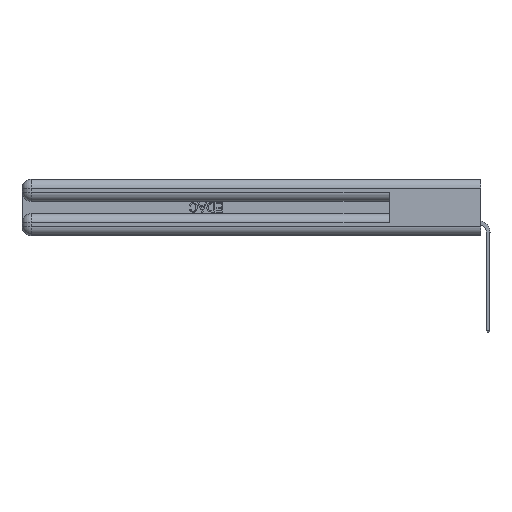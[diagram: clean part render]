
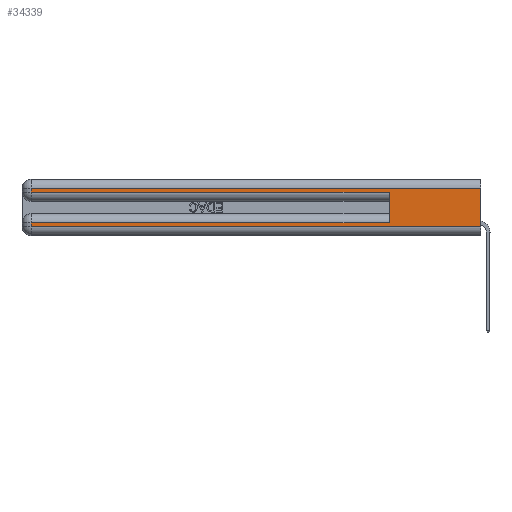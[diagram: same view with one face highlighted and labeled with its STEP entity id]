
A CAD part, left-side view. The second image highlights one B-rep face of the part: STEP entity #34339.
In plain terms, the highlighted planar face has unit normal (-1, 0, 0).
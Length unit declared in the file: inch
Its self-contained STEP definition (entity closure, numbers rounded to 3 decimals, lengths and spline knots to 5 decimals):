
#179 = VECTOR ( 'NONE', #30480, 39.37008 ) ;
#824 = CARTESIAN_POINT ( 'NONE',  ( 0., 2.94, 0.37 ) ) ;
#914 = CARTESIAN_POINT ( 'NONE',  ( 0., 0.6, 0.085 ) ) ;
#1664 = CARTESIAN_POINT ( 'NONE',  ( 0., 0., 0.31 ) ) ;
#2290 = EDGE_CURVE ( 'NONE', #16596, #33285, #25107, .T. ) ;
#2438 = VECTOR ( 'NONE', #9605, 39.37008 ) ;
#3747 = LINE ( 'NONE', #824, #2438 ) ;
#3851 = CARTESIAN_POINT ( 'NONE',  ( 0., 2.94, 0.37 ) ) ;
#4039 = DIRECTION ( 'NONE',  ( 0., 0., -1. ) ) ;
#4393 = FACE_OUTER_BOUND ( 'NONE', #9699, .T. ) ;
#5844 = ORIENTED_EDGE ( 'NONE', *, *, #26525, .F. ) ;
#5967 = CARTESIAN_POINT ( 'NONE',  ( 0., 2.94, 0.285 ) ) ;
#6519 = VERTEX_POINT ( 'NONE', #26959 ) ;
#6726 = DIRECTION ( 'NONE',  ( 0., 0., -1. ) ) ;
#8033 = CARTESIAN_POINT ( 'NONE',  ( 0., 2.94, 0.31 ) ) ;
#8078 = VECTOR ( 'NONE', #27937, 39.37008 ) ;
#8885 = ORIENTED_EDGE ( 'NONE', *, *, #13272, .T. ) ;
#9605 = DIRECTION ( 'NONE',  ( 0., 0., -1. ) ) ;
#9699 = EDGE_LOOP ( 'NONE', ( #5844, #21100, #18361, #8885, #35085, #35553, #29935, #29066 ) ) ;
#10263 = VERTEX_POINT ( 'NONE', #914 ) ;
#10519 = VERTEX_POINT ( 'NONE', #1664 ) ;
#11010 = EDGE_CURVE ( 'NONE', #10519, #34009, #36066, .T. ) ;
#12023 = CARTESIAN_POINT ( 'NONE',  ( 0., 0., 0.37 ) ) ;
#13272 = EDGE_CURVE ( 'NONE', #28745, #6519, #24202, .T. ) ;
#14786 = CARTESIAN_POINT ( 'NONE',  ( 0., 0., 0.31 ) ) ;
#16596 = VERTEX_POINT ( 'NONE', #36293 ) ;
#18361 = ORIENTED_EDGE ( 'NONE', *, *, #22460, .T. ) ;
#18586 = CARTESIAN_POINT ( 'NONE',  ( 0., 0., 0.37 ) ) ;
#18626 = DIRECTION ( 'NONE',  ( 0., -1., 0. ) ) ;
#18741 = VECTOR ( 'NONE', #4039, 39.37008 ) ;
#18929 = LINE ( 'NONE', #27494, #179 ) ;
#19110 = EDGE_CURVE ( 'NONE', #10263, #6519, #18929, .T. ) ;
#21100 = ORIENTED_EDGE ( 'NONE', *, *, #11010, .T. ) ;
#22460 = EDGE_CURVE ( 'NONE', #34009, #28745, #29894, .T. ) ;
#23153 = DIRECTION ( 'NONE',  ( 0., 1., 0. ) ) ;
#23693 = VECTOR ( 'NONE', #23153, 39.37008 ) ;
#24146 = VECTOR ( 'NONE', #27720, 39.37008 ) ;
#24202 = LINE ( 'NONE', #24637, #38742 ) ;
#24637 = CARTESIAN_POINT ( 'NONE',  ( 0., 0., 0.285 ) ) ;
#25107 = LINE ( 'NONE', #33720, #24146 ) ;
#26525 = EDGE_CURVE ( 'NONE', #10519, #33285, #26722, .T. ) ;
#26722 = LINE ( 'NONE', #18586, #18741 ) ;
#26899 = CARTESIAN_POINT ( 'NONE',  ( 0., 2.94, 0.085 ) ) ;
#26959 = CARTESIAN_POINT ( 'NONE',  ( 0., 0.6, 0.285 ) ) ;
#27494 = CARTESIAN_POINT ( 'NONE',  ( 0., 0.6, 0.145 ) ) ;
#27720 = DIRECTION ( 'NONE',  ( 0., -1., 0. ) ) ;
#27937 = DIRECTION ( 'NONE',  ( 0., 1., 0. ) ) ;
#28745 = VERTEX_POINT ( 'NONE', #5967 ) ;
#29066 = ORIENTED_EDGE ( 'NONE', *, *, #2290, .T. ) ;
#29894 = LINE ( 'NONE', #3851, #35963 ) ;
#29935 = ORIENTED_EDGE ( 'NONE', *, *, #35843, .T. ) ;
#30027 = DIRECTION ( 'NONE',  ( 1., 0., 0. ) ) ;
#30480 = DIRECTION ( 'NONE',  ( 0., 0., 1. ) ) ;
#31389 = AXIS2_PLACEMENT_3D ( 'NONE', #12023, #30027, #33038 ) ;
#32585 = LINE ( 'NONE', #35015, #23693 ) ;
#33014 = EDGE_CURVE ( 'NONE', #10263, #35706, #32585, .T. ) ;
#33038 = DIRECTION ( 'NONE',  ( 0., 0., -1. ) ) ;
#33285 = VERTEX_POINT ( 'NONE', #36793 ) ;
#33720 = CARTESIAN_POINT ( 'NONE',  ( 0., 0., 0.06 ) ) ;
#34009 = VERTEX_POINT ( 'NONE', #8033 ) ;
#34339 = ADVANCED_FACE ( 'NONE', ( #4393 ), #38584, .F. ) ;
#35015 = CARTESIAN_POINT ( 'NONE',  ( 0., 0., 0.085 ) ) ;
#35085 = ORIENTED_EDGE ( 'NONE', *, *, #19110, .F. ) ;
#35553 = ORIENTED_EDGE ( 'NONE', *, *, #33014, .T. ) ;
#35706 = VERTEX_POINT ( 'NONE', #26899 ) ;
#35843 = EDGE_CURVE ( 'NONE', #35706, #16596, #3747, .T. ) ;
#35963 = VECTOR ( 'NONE', #6726, 39.37008 ) ;
#36066 = LINE ( 'NONE', #14786, #8078 ) ;
#36293 = CARTESIAN_POINT ( 'NONE',  ( 0., 2.94, 0.06 ) ) ;
#36793 = CARTESIAN_POINT ( 'NONE',  ( 0., 0., 0.06 ) ) ;
#38584 = PLANE ( 'NONE',  #31389 ) ;
#38742 = VECTOR ( 'NONE', #18626, 39.37008 ) ;
